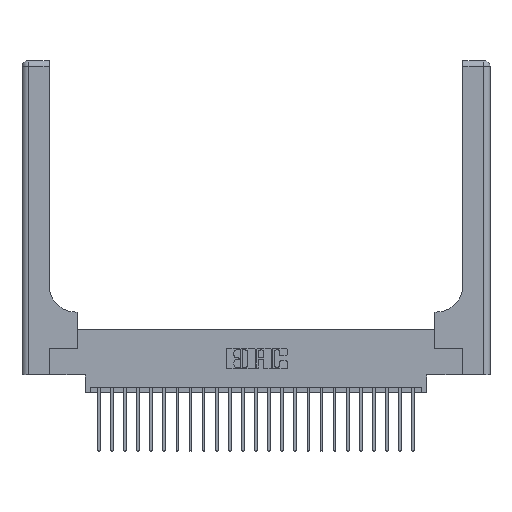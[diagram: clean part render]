
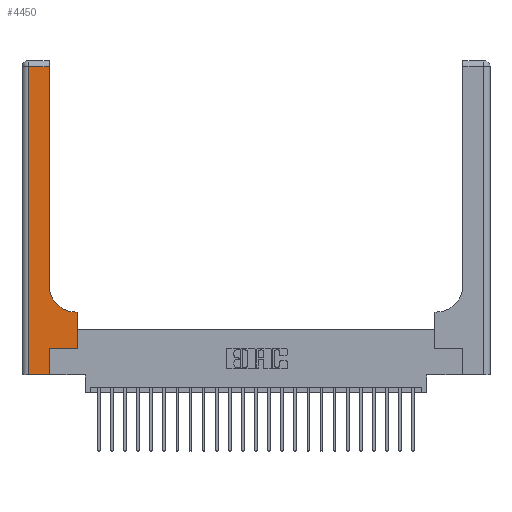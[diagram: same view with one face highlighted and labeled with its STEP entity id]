
A CAD part, top view. The second image highlights one B-rep face of the part: STEP entity #4450.
In plain terms, the highlighted planar face has unit normal (0, 0, 1).
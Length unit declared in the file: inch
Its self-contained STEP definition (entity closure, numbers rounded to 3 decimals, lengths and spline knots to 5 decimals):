
#22 = EDGE_CURVE ( 'NONE', #15853, #15130, #3912, .T. ) ;
#287 = VERTEX_POINT ( 'NONE', #3752 ) ;
#380 = LINE ( 'NONE', #2444, #20079 ) ;
#730 = CARTESIAN_POINT ( 'NONE',  ( 0.26, 0.6, 0.37 ) ) ;
#899 = CARTESIAN_POINT ( 'NONE',  ( 0.528, 0.25, 0.37 ) ) ;
#1698 = CARTESIAN_POINT ( 'NONE',  ( 0.06, 0., 0.37 ) ) ;
#1905 = DIRECTION ( 'NONE',  ( 0., 0., -1. ) ) ;
#1995 = DIRECTION ( 'NONE',  ( 0., 1., 0. ) ) ;
#2427 = ORIENTED_EDGE ( 'NONE', *, *, #16145, .T. ) ;
#2444 = CARTESIAN_POINT ( 'NONE',  ( 0., 2.94, 0.37 ) ) ;
#2768 = DIRECTION ( 'NONE',  ( 1., 0., 0. ) ) ;
#3720 = EDGE_CURVE ( 'NONE', #15130, #287, #12132, .T. ) ;
#3752 = CARTESIAN_POINT ( 'NONE',  ( 0.528, 0.6, 0.37 ) ) ;
#3912 = LINE ( 'NONE', #7436, #22907 ) ;
#3942 = AXIS2_PLACEMENT_3D ( 'NONE', #7296, #20067, #9161 ) ;
#4450 = ADVANCED_FACE ( 'NONE', ( #19190 ), #14868, .F. ) ;
#4691 = EDGE_CURVE ( 'NONE', #287, #13772, #5997, .T. ) ;
#4695 = DIRECTION ( 'NONE',  ( 0., 1., 0. ) ) ;
#4857 = ORIENTED_EDGE ( 'NONE', *, *, #12343, .T. ) ;
#5430 = ORIENTED_EDGE ( 'NONE', *, *, #7999, .T. ) ;
#5938 = CARTESIAN_POINT ( 'NONE',  ( 0.51, 0.6, 0.37 ) ) ;
#5997 = LINE ( 'NONE', #730, #10375 ) ;
#7296 = CARTESIAN_POINT ( 'NONE',  ( 0.51, 0.85, 0.37 ) ) ;
#7397 = VECTOR ( 'NONE', #15442, 39.37008 ) ;
#7436 = CARTESIAN_POINT ( 'NONE',  ( 0.265, 0.25, 0.37 ) ) ;
#7452 = DIRECTION ( 'NONE',  ( 1., 0., 0. ) ) ;
#7570 = VERTEX_POINT ( 'NONE', #1698 ) ;
#7999 = EDGE_CURVE ( 'NONE', #7570, #14769, #19363, .T. ) ;
#9161 = DIRECTION ( 'NONE',  ( 1., 0., 0. ) ) ;
#9891 = EDGE_CURVE ( 'NONE', #15149, #16678, #380, .T. ) ;
#10375 = VECTOR ( 'NONE', #13816, 39.37008 ) ;
#12132 = LINE ( 'NONE', #899, #16974 ) ;
#12343 = EDGE_CURVE ( 'NONE', #16678, #7570, #17138, .T. ) ;
#13255 = ORIENTED_EDGE ( 'NONE', *, *, #4691, .T. ) ;
#13260 = CARTESIAN_POINT ( 'NONE',  ( 0.265, 0., 0.37 ) ) ;
#13610 = CARTESIAN_POINT ( 'NONE',  ( 0.06, 3., 0.37 ) ) ;
#13772 = VERTEX_POINT ( 'NONE', #5938 ) ;
#13794 = CARTESIAN_POINT ( 'NONE',  ( 0.26, 2.94, 0.37 ) ) ;
#13816 = DIRECTION ( 'NONE',  ( -1., 0., 0. ) ) ;
#13974 = DIRECTION ( 'NONE',  ( 0., 1., 0. ) ) ;
#14769 = VERTEX_POINT ( 'NONE', #16297 ) ;
#14798 = EDGE_CURVE ( 'NONE', #13772, #18897, #17342, .T. ) ;
#14868 = PLANE ( 'NONE',  #19846 ) ;
#14942 = DIRECTION ( 'NONE',  ( -1., 0., 0. ) ) ;
#15130 = VERTEX_POINT ( 'NONE', #19094 ) ;
#15149 = VERTEX_POINT ( 'NONE', #13794 ) ;
#15250 = ORIENTED_EDGE ( 'NONE', *, *, #16593, .T. ) ;
#15442 = DIRECTION ( 'NONE',  ( 0., -1., 0. ) ) ;
#15467 = DIRECTION ( 'NONE',  ( -1., 0., 0. ) ) ;
#15800 = VECTOR ( 'NONE', #1995, 39.37008 ) ;
#15830 = ORIENTED_EDGE ( 'NONE', *, *, #22, .T. ) ;
#15853 = VERTEX_POINT ( 'NONE', #18373 ) ;
#16145 = EDGE_CURVE ( 'NONE', #18897, #15149, #18417, .T. ) ;
#16297 = CARTESIAN_POINT ( 'NONE',  ( 0.265, 0., 0.37 ) ) ;
#16593 = EDGE_CURVE ( 'NONE', #14769, #15853, #20590, .T. ) ;
#16678 = VERTEX_POINT ( 'NONE', #22557 ) ;
#16951 = ORIENTED_EDGE ( 'NONE', *, *, #3720, .T. ) ;
#16974 = VECTOR ( 'NONE', #13974, 39.37008 ) ;
#17138 = LINE ( 'NONE', #13610, #7397 ) ;
#17342 = CIRCLE ( 'NONE', #3942, 0.25 ) ;
#17493 = CARTESIAN_POINT ( 'NONE',  ( 0., 0., 0.37 ) ) ;
#17573 = CARTESIAN_POINT ( 'NONE',  ( 0.26, 3., 0.37 ) ) ;
#18343 = CARTESIAN_POINT ( 'NONE',  ( 0., 3., 0.37 ) ) ;
#18373 = CARTESIAN_POINT ( 'NONE',  ( 0.265, 0.25, 0.37 ) ) ;
#18417 = LINE ( 'NONE', #17573, #23270 ) ;
#18897 = VERTEX_POINT ( 'NONE', #22757 ) ;
#18912 = ORIENTED_EDGE ( 'NONE', *, *, #9891, .T. ) ;
#19094 = CARTESIAN_POINT ( 'NONE',  ( 0.528, 0.25, 0.37 ) ) ;
#19190 = FACE_OUTER_BOUND ( 'NONE', #23572, .T. ) ;
#19363 = LINE ( 'NONE', #17493, #23656 ) ;
#19846 = AXIS2_PLACEMENT_3D ( 'NONE', #18343, #1905, #14942 ) ;
#20067 = DIRECTION ( 'NONE',  ( 0., 0., -1. ) ) ;
#20079 = VECTOR ( 'NONE', #15467, 39.37008 ) ;
#20590 = LINE ( 'NONE', #13260, #15800 ) ;
#22557 = CARTESIAN_POINT ( 'NONE',  ( 0.06, 2.94, 0.37 ) ) ;
#22757 = CARTESIAN_POINT ( 'NONE',  ( 0.26, 0.85, 0.37 ) ) ;
#22907 = VECTOR ( 'NONE', #7452, 39.37008 ) ;
#22932 = ORIENTED_EDGE ( 'NONE', *, *, #14798, .T. ) ;
#23270 = VECTOR ( 'NONE', #4695, 39.37008 ) ;
#23572 = EDGE_LOOP ( 'NONE', ( #2427, #18912, #4857, #5430, #15250, #15830, #16951, #13255, #22932 ) ) ;
#23656 = VECTOR ( 'NONE', #2768, 39.37008 ) ;
